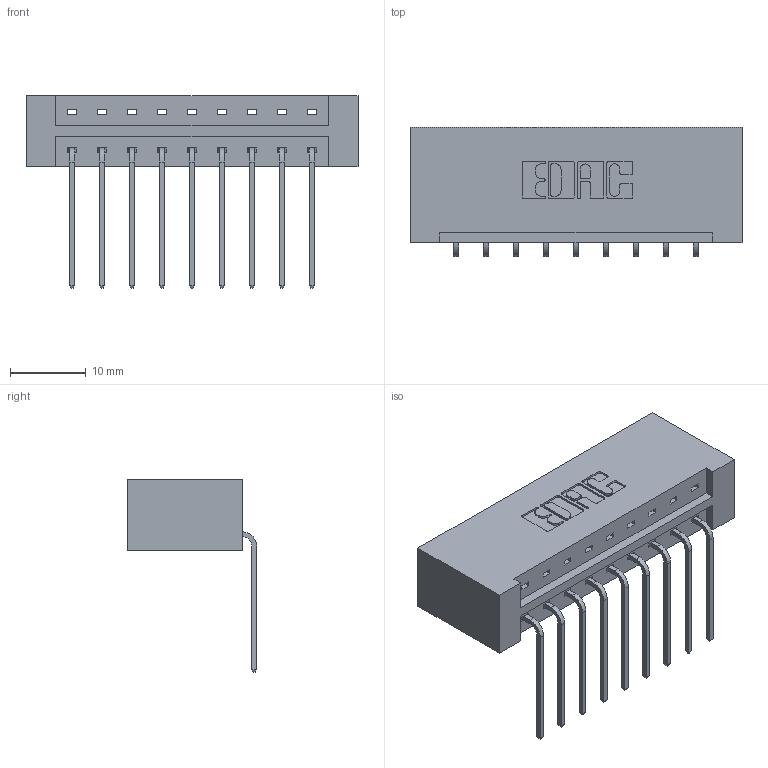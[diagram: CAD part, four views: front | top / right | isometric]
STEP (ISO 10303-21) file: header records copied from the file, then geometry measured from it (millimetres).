
FILE_DESCRIPTION (( 'STEP AP203' ), '1' );
FILE_NAME ('833-009-559-101.STEP', '2020-05-30T17:50:15', ( '' ), ( '' ), 'SwSTEP 2.0', 'SolidWorks 2020', '' );
FILE_SCHEMA (( 'CONFIG_CONTROL_DESIGN' ));
Length unit declared in the file: inch
Products named in the file (3): 345-292-001_558 559 Tail - 1; 833 Part_Lugless; 833-009-559-101
Assembly tree (10 placements, depth 2):
  833-009-559-101
    833 Part_Lugless
    345-292-001_558 559 Tail - 1  x9
Bounding box: 43.92 x 17.09 x 25.53 mm (x, y, z)
Volume: 4778.2 mm3; surface area: 5094.3 mm2
Topology: 10 solids, 10 shells, 646 faces, 1925 edges, 1270 vertices
Faces by surface type: plane 462, cylinder 184
Entity records: 9577 total; most frequent: CARTESIAN_POINT 1665, ORIENTED_EDGE 1610, DIRECTION 1463, EDGE_CURVE 805, LINE 685, VECTOR 685, VERTEX_POINT 534, AXIS2_PLACEMENT_3D 389
